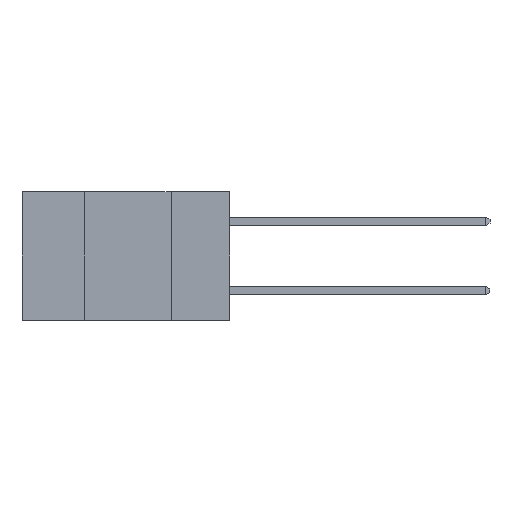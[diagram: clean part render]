
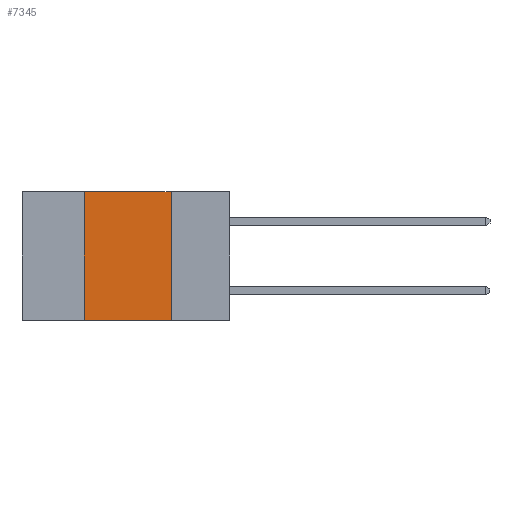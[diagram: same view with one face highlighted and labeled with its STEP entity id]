
A CAD part, left-side view. The second image highlights one B-rep face of the part: STEP entity #7345.
In plain terms, the highlighted planar face has unit normal (-1, 0, 0).
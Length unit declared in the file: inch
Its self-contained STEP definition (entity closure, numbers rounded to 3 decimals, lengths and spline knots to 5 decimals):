
#404 = ORIENTED_EDGE ( 'NONE', *, *, #10691, .F. ) ;
#422 = DIRECTION ( 'NONE',  ( 0., -1., 0. ) ) ;
#465 = CARTESIAN_POINT ( 'NONE',  ( 0., 0.6, 0. ) ) ;
#682 = LINE ( 'NONE', #2988, #2642 ) ;
#791 = LINE ( 'NONE', #2587, #5570 ) ;
#1163 = AXIS2_PLACEMENT_3D ( 'NONE', #9263, #2689, #8171 ) ;
#1318 = DIRECTION ( 'NONE',  ( 0., 0., 1. ) ) ;
#1372 = VERTEX_POINT ( 'NONE', #9208 ) ;
#1409 = CARTESIAN_POINT ( 'NONE',  ( 0., 0.42, 0. ) ) ;
#1763 = VERTEX_POINT ( 'NONE', #3220 ) ;
#2293 = VECTOR ( 'NONE', #1318, 39.37008 ) ;
#2411 = VERTEX_POINT ( 'NONE', #8877 ) ;
#2518 = VECTOR ( 'NONE', #422, 39.37008 ) ;
#2587 = CARTESIAN_POINT ( 'NONE',  ( 0., 0.6, -0.37 ) ) ;
#2590 = CARTESIAN_POINT ( 'NONE',  ( 0., 0.42, 0. ) ) ;
#2642 = VECTOR ( 'NONE', #6404, 39.37008 ) ;
#2689 = DIRECTION ( 'NONE',  ( 1., 0., 0. ) ) ;
#2948 = ORIENTED_EDGE ( 'NONE', *, *, #4958, .F. ) ;
#2988 = CARTESIAN_POINT ( 'NONE',  ( 0., 0.17, 0. ) ) ;
#3220 = CARTESIAN_POINT ( 'NONE',  ( 0., 0.17, 0. ) ) ;
#4123 = DIRECTION ( 'NONE',  ( 0., -1., 0. ) ) ;
#4958 = EDGE_CURVE ( 'NONE', #1763, #2411, #682, .T. ) ;
#5196 = VERTEX_POINT ( 'NONE', #2590 ) ;
#5510 = ORIENTED_EDGE ( 'NONE', *, *, #7251, .F. ) ;
#5570 = VECTOR ( 'NONE', #4123, 39.37008 ) ;
#6178 = PLANE ( 'NONE',  #1163 ) ;
#6404 = DIRECTION ( 'NONE',  ( 0., 0., -1. ) ) ;
#6711 = ORIENTED_EDGE ( 'NONE', *, *, #7585, .T. ) ;
#7251 = EDGE_CURVE ( 'NONE', #1372, #5196, #11225, .T. ) ;
#7345 = ADVANCED_FACE ( 'NONE', ( #8540 ), #6178, .F. ) ;
#7585 = EDGE_CURVE ( 'NONE', #1372, #2411, #791, .T. ) ;
#8171 = DIRECTION ( 'NONE',  ( 0., 0., -1. ) ) ;
#8540 = FACE_OUTER_BOUND ( 'NONE', #9001, .T. ) ;
#8877 = CARTESIAN_POINT ( 'NONE',  ( 0., 0.17, -0.37 ) ) ;
#9001 = EDGE_LOOP ( 'NONE', ( #2948, #404, #5510, #6711 ) ) ;
#9208 = CARTESIAN_POINT ( 'NONE',  ( 0., 0.42, -0.37 ) ) ;
#9263 = CARTESIAN_POINT ( 'NONE',  ( 0., 0.6, 0. ) ) ;
#9763 = LINE ( 'NONE', #465, #2518 ) ;
#10691 = EDGE_CURVE ( 'NONE', #5196, #1763, #9763, .T. ) ;
#11225 = LINE ( 'NONE', #1409, #2293 ) ;
